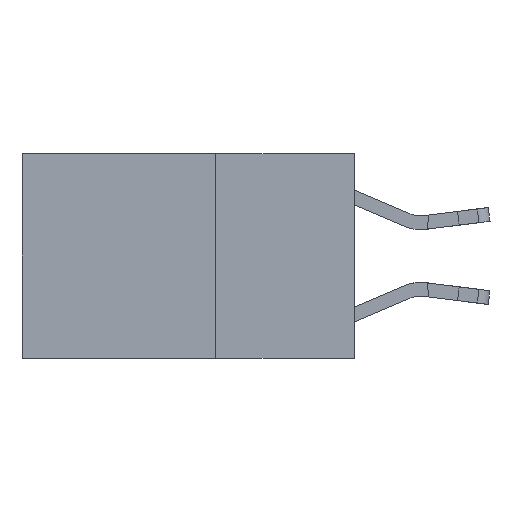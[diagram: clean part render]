
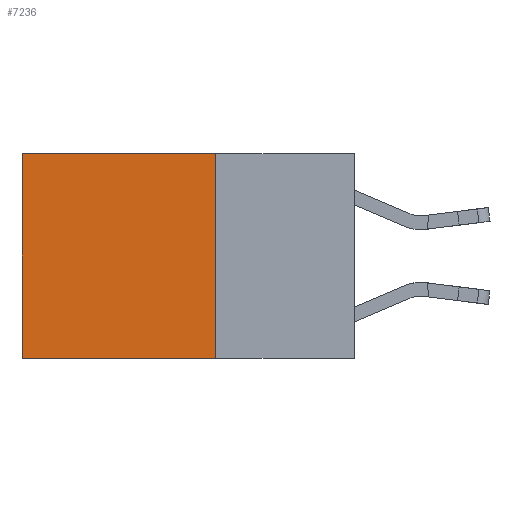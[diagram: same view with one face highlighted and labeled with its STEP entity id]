
A CAD part, left-side view. The second image highlights one B-rep face of the part: STEP entity #7236.
In plain terms, the highlighted planar face has unit normal (-1, 0, 0).
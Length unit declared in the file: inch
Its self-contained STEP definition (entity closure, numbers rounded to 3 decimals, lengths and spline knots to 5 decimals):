
#117 = PLANE ( 'NONE',  #3533 ) ;
#948 = CARTESIAN_POINT ( 'NONE',  ( 0.2625, 0.6, 0. ) ) ;
#1126 = VERTEX_POINT ( 'NONE', #948 ) ;
#1241 = DIRECTION ( 'NONE',  ( 0., 0., -1. ) ) ;
#2354 = ORIENTED_EDGE ( 'NONE', *, *, #13371, .F. ) ;
#2400 = CARTESIAN_POINT ( 'NONE',  ( 0.2625, 0.25, -0.37 ) ) ;
#2595 = LINE ( 'NONE', #3570, #11694 ) ;
#2716 = DIRECTION ( 'NONE',  ( 0., 1., 0. ) ) ;
#3233 = CARTESIAN_POINT ( 'NONE',  ( 0.2625, 0.25, 0. ) ) ;
#3533 = AXIS2_PLACEMENT_3D ( 'NONE', #5709, #7945, #1241 ) ;
#3570 = CARTESIAN_POINT ( 'NONE',  ( 0.2625, 0.6, 0. ) ) ;
#4717 = EDGE_CURVE ( 'NONE', #7246, #7597, #6102, .T. ) ;
#4864 = CARTESIAN_POINT ( 'NONE',  ( 0.2625, 0.25, 0. ) ) ;
#5300 = ORIENTED_EDGE ( 'NONE', *, *, #11421, .T. ) ;
#5687 = DIRECTION ( 'NONE',  ( 0., 1., 0. ) ) ;
#5709 = CARTESIAN_POINT ( 'NONE',  ( 0.2625, 0.25, 0. ) ) ;
#5723 = VECTOR ( 'NONE', #11418, 39.37008 ) ;
#6102 = LINE ( 'NONE', #6764, #11553 ) ;
#6190 = VECTOR ( 'NONE', #2716, 39.37008 ) ;
#6299 = FACE_OUTER_BOUND ( 'NONE', #13234, .T. ) ;
#6764 = CARTESIAN_POINT ( 'NONE',  ( 0.2625, 0.25, -0.37 ) ) ;
#7236 = ADVANCED_FACE ( 'NONE', ( #6299 ), #117, .F. ) ;
#7246 = VERTEX_POINT ( 'NONE', #2400 ) ;
#7597 = VERTEX_POINT ( 'NONE', #8643 ) ;
#7921 = ORIENTED_EDGE ( 'NONE', *, *, #12586, .T. ) ;
#7945 = DIRECTION ( 'NONE',  ( 1., 0., 0. ) ) ;
#8643 = CARTESIAN_POINT ( 'NONE',  ( 0.2625, 0.6, -0.37 ) ) ;
#8661 = LINE ( 'NONE', #4864, #5723 ) ;
#9124 = LINE ( 'NONE', #13665, #6190 ) ;
#10381 = VERTEX_POINT ( 'NONE', #3233 ) ;
#10794 = ORIENTED_EDGE ( 'NONE', *, *, #4717, .F. ) ;
#11252 = DIRECTION ( 'NONE',  ( 0., 0., -1. ) ) ;
#11418 = DIRECTION ( 'NONE',  ( 0., 0., -1. ) ) ;
#11421 = EDGE_CURVE ( 'NONE', #10381, #1126, #9124, .T. ) ;
#11553 = VECTOR ( 'NONE', #5687, 39.37008 ) ;
#11694 = VECTOR ( 'NONE', #11252, 39.37008 ) ;
#12586 = EDGE_CURVE ( 'NONE', #1126, #7597, #2595, .T. ) ;
#13234 = EDGE_LOOP ( 'NONE', ( #7921, #10794, #2354, #5300 ) ) ;
#13371 = EDGE_CURVE ( 'NONE', #10381, #7246, #8661, .T. ) ;
#13665 = CARTESIAN_POINT ( 'NONE',  ( 0.2625, 0.25, 0. ) ) ;
